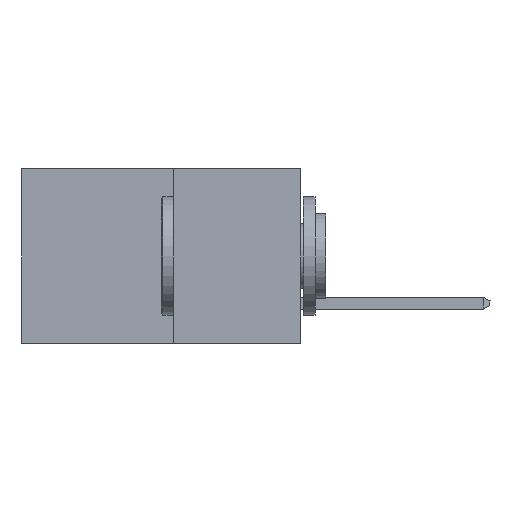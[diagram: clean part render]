
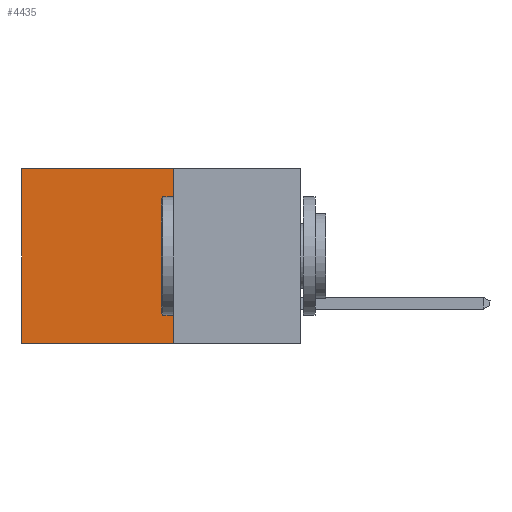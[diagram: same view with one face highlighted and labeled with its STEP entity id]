
A CAD part, left-side view. The second image highlights one B-rep face of the part: STEP entity #4435.
In plain terms, the highlighted planar face has unit normal (-1, 0, 0).
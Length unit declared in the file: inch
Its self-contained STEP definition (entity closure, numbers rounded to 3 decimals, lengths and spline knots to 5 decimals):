
#620 = EDGE_LOOP ( 'NONE', ( #7378, #20229, #4201, #7986 ) ) ;
#1296 = EDGE_CURVE ( 'NONE', #14679, #12940, #23164, .T. ) ;
#1498 = DIRECTION ( 'NONE',  ( 0., 1., 0. ) ) ;
#1679 = EDGE_CURVE ( 'NONE', #14679, #4985, #9000, .T. ) ;
#2683 = DIRECTION ( 'NONE',  ( 0., 0., -1. ) ) ;
#4201 = ORIENTED_EDGE ( 'NONE', *, *, #1679, .F. ) ;
#4435 = ADVANCED_FACE ( 'NONE', ( #7929 ), #21466, .F. ) ;
#4985 = VERTEX_POINT ( 'NONE', #23733 ) ;
#5786 = LINE ( 'NONE', #25410, #24029 ) ;
#6817 = AXIS2_PLACEMENT_3D ( 'NONE', #20708, #19688, #19602 ) ;
#7077 = VECTOR ( 'NONE', #1498, 39.37008 ) ;
#7378 = ORIENTED_EDGE ( 'NONE', *, *, #25876, .T. ) ;
#7929 = FACE_OUTER_BOUND ( 'NONE', #620, .T. ) ;
#7986 = ORIENTED_EDGE ( 'NONE', *, *, #1296, .T. ) ;
#9000 = LINE ( 'NONE', #12199, #24387 ) ;
#12199 = CARTESIAN_POINT ( 'NONE',  ( 0.277, 0.27, -0.37 ) ) ;
#12940 = VERTEX_POINT ( 'NONE', #18530 ) ;
#13934 = DIRECTION ( 'NONE',  ( 0., 1., 0. ) ) ;
#14679 = VERTEX_POINT ( 'NONE', #22648 ) ;
#15519 = DIRECTION ( 'NONE',  ( 0., 0., -1. ) ) ;
#17840 = VECTOR ( 'NONE', #13934, 39.37008 ) ;
#18530 = CARTESIAN_POINT ( 'NONE',  ( 0.277, 0.59, 0. ) ) ;
#19602 = DIRECTION ( 'NONE',  ( 0., 0., -1. ) ) ;
#19688 = DIRECTION ( 'NONE',  ( 1., 0., 0. ) ) ;
#20229 = ORIENTED_EDGE ( 'NONE', *, *, #25473, .F. ) ;
#20350 = VERTEX_POINT ( 'NONE', #23172 ) ;
#20708 = CARTESIAN_POINT ( 'NONE',  ( 0.277, 0.27, -0.37 ) ) ;
#21466 = PLANE ( 'NONE',  #6817 ) ;
#22648 = CARTESIAN_POINT ( 'NONE',  ( 0.277, 0.27, 0. ) ) ;
#23075 = LINE ( 'NONE', #23878, #17840 ) ;
#23164 = LINE ( 'NONE', #23286, #7077 ) ;
#23172 = CARTESIAN_POINT ( 'NONE',  ( 0.277, 0.59, -0.37 ) ) ;
#23286 = CARTESIAN_POINT ( 'NONE',  ( 0.277, 0.27, 0. ) ) ;
#23733 = CARTESIAN_POINT ( 'NONE',  ( 0.277, 0.27, -0.37 ) ) ;
#23878 = CARTESIAN_POINT ( 'NONE',  ( 0.277, 0.27, -0.37 ) ) ;
#24029 = VECTOR ( 'NONE', #15519, 39.37008 ) ;
#24387 = VECTOR ( 'NONE', #2683, 39.37008 ) ;
#25410 = CARTESIAN_POINT ( 'NONE',  ( 0.277, 0.59, -0.37 ) ) ;
#25473 = EDGE_CURVE ( 'NONE', #4985, #20350, #23075, .T. ) ;
#25876 = EDGE_CURVE ( 'NONE', #12940, #20350, #5786, .T. ) ;
